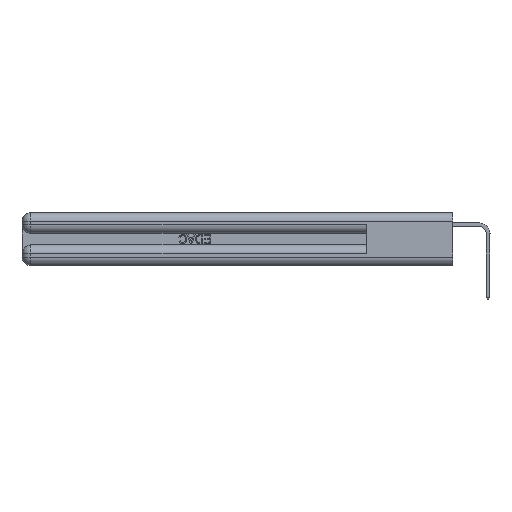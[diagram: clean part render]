
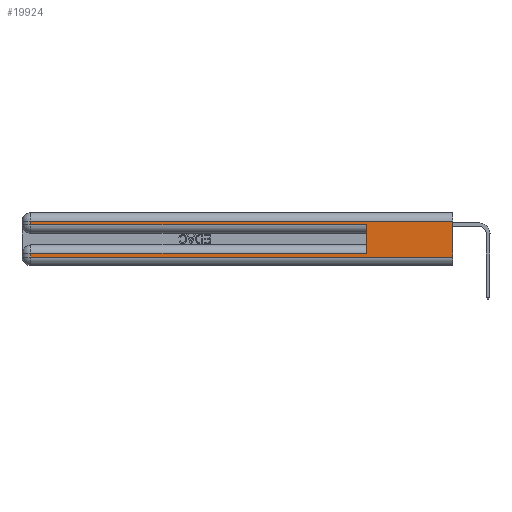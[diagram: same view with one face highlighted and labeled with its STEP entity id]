
A CAD part, left-side view. The second image highlights one B-rep face of the part: STEP entity #19924.
In plain terms, the highlighted planar face has unit normal (-1, 0, 0).
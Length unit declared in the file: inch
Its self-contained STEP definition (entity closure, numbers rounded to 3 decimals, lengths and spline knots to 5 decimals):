
#192 = VERTEX_POINT ( 'NONE', #7704 ) ;
#294 = DIRECTION ( 'NONE',  ( 0., -1., 0. ) ) ;
#431 = ORIENTED_EDGE ( 'NONE', *, *, #45958, .T. ) ;
#3605 = LINE ( 'NONE', #41046, #41292 ) ;
#4216 = CARTESIAN_POINT ( 'NONE',  ( 0., 2.94, 0.31 ) ) ;
#6360 = CARTESIAN_POINT ( 'NONE',  ( 0., 2.94, 0.37 ) ) ;
#6785 = EDGE_CURVE ( 'NONE', #33862, #33027, #36483, .T. ) ;
#7072 = VECTOR ( 'NONE', #30509, 39.37008 ) ;
#7704 = CARTESIAN_POINT ( 'NONE',  ( 0., 0.6, 0.085 ) ) ;
#7809 = CARTESIAN_POINT ( 'NONE',  ( 0., 2.94, 0.285 ) ) ;
#8069 = EDGE_CURVE ( 'NONE', #15839, #33027, #28467, .T. ) ;
#8267 = PLANE ( 'NONE',  #28253 ) ;
#11405 = FACE_OUTER_BOUND ( 'NONE', #26347, .T. ) ;
#11477 = EDGE_CURVE ( 'NONE', #33862, #34792, #3605, .T. ) ;
#11959 = DIRECTION ( 'NONE',  ( 1., 0., 0. ) ) ;
#12282 = EDGE_CURVE ( 'NONE', #23848, #15839, #26407, .T. ) ;
#12825 = CARTESIAN_POINT ( 'NONE',  ( 0., 2.94, 0.085 ) ) ;
#15839 = VERTEX_POINT ( 'NONE', #47384 ) ;
#17404 = EDGE_CURVE ( 'NONE', #192, #23848, #44761, .T. ) ;
#17557 = DIRECTION ( 'NONE',  ( 0., 0., -1. ) ) ;
#18481 = CARTESIAN_POINT ( 'NONE',  ( 0., 0., 0.06 ) ) ;
#19889 = CARTESIAN_POINT ( 'NONE',  ( 0., 2.94, 0.37 ) ) ;
#19924 = ADVANCED_FACE ( 'NONE', ( #11405 ), #8267, .F. ) ;
#20676 = ORIENTED_EDGE ( 'NONE', *, *, #12282, .T. ) ;
#21058 = VERTEX_POINT ( 'NONE', #7809 ) ;
#21318 = CARTESIAN_POINT ( 'NONE',  ( 0., 0., 0.06 ) ) ;
#21478 = DIRECTION ( 'NONE',  ( 0., -1., 0. ) ) ;
#21936 = EDGE_CURVE ( 'NONE', #192, #43079, #38016, .T. ) ;
#23221 = CARTESIAN_POINT ( 'NONE',  ( 0., 0., 0.085 ) ) ;
#23436 = DIRECTION ( 'NONE',  ( 0., 0., -1. ) ) ;
#23437 = ORIENTED_EDGE ( 'NONE', *, *, #28174, .T. ) ;
#23848 = VERTEX_POINT ( 'NONE', #12825 ) ;
#24552 = DIRECTION ( 'NONE',  ( 0., 0., 1. ) ) ;
#25631 = LINE ( 'NONE', #19889, #26745 ) ;
#26347 = EDGE_LOOP ( 'NONE', ( #36931, #46197, #23437, #431, #42446, #27129, #20676, #36000 ) ) ;
#26407 = LINE ( 'NONE', #6360, #44652 ) ;
#26550 = DIRECTION ( 'NONE',  ( 0., 1., 0. ) ) ;
#26745 = VECTOR ( 'NONE', #23436, 39.37008 ) ;
#27129 = ORIENTED_EDGE ( 'NONE', *, *, #17404, .T. ) ;
#27294 = VECTOR ( 'NONE', #21478, 39.37008 ) ;
#28174 = EDGE_CURVE ( 'NONE', #34792, #21058, #25631, .T. ) ;
#28253 = AXIS2_PLACEMENT_3D ( 'NONE', #33844, #11959, #37500 ) ;
#28329 = VECTOR ( 'NONE', #24552, 39.37008 ) ;
#28452 = VECTOR ( 'NONE', #294, 39.37008 ) ;
#28467 = LINE ( 'NONE', #21318, #27294 ) ;
#29569 = LINE ( 'NONE', #44083, #28452 ) ;
#30509 = DIRECTION ( 'NONE',  ( 0., 1., 0. ) ) ;
#33027 = VERTEX_POINT ( 'NONE', #18481 ) ;
#33844 = CARTESIAN_POINT ( 'NONE',  ( 0., 0., 0.37 ) ) ;
#33862 = VERTEX_POINT ( 'NONE', #35009 ) ;
#34792 = VERTEX_POINT ( 'NONE', #4216 ) ;
#35009 = CARTESIAN_POINT ( 'NONE',  ( 0., 0., 0.31 ) ) ;
#35538 = DIRECTION ( 'NONE',  ( 0., 0., -1. ) ) ;
#36000 = ORIENTED_EDGE ( 'NONE', *, *, #8069, .T. ) ;
#36483 = LINE ( 'NONE', #46371, #46183 ) ;
#36931 = ORIENTED_EDGE ( 'NONE', *, *, #6785, .F. ) ;
#37500 = DIRECTION ( 'NONE',  ( 0., 0., -1. ) ) ;
#38016 = LINE ( 'NONE', #39034, #28329 ) ;
#39034 = CARTESIAN_POINT ( 'NONE',  ( 0., 0.6, 0.145 ) ) ;
#41046 = CARTESIAN_POINT ( 'NONE',  ( 0., 0., 0.31 ) ) ;
#41292 = VECTOR ( 'NONE', #26550, 39.37008 ) ;
#42446 = ORIENTED_EDGE ( 'NONE', *, *, #21936, .F. ) ;
#43009 = CARTESIAN_POINT ( 'NONE',  ( 0., 0.6, 0.285 ) ) ;
#43079 = VERTEX_POINT ( 'NONE', #43009 ) ;
#44083 = CARTESIAN_POINT ( 'NONE',  ( 0., 0., 0.285 ) ) ;
#44652 = VECTOR ( 'NONE', #17557, 39.37008 ) ;
#44761 = LINE ( 'NONE', #23221, #7072 ) ;
#45958 = EDGE_CURVE ( 'NONE', #21058, #43079, #29569, .T. ) ;
#46183 = VECTOR ( 'NONE', #35538, 39.37008 ) ;
#46197 = ORIENTED_EDGE ( 'NONE', *, *, #11477, .T. ) ;
#46371 = CARTESIAN_POINT ( 'NONE',  ( 0., 0., 0.37 ) ) ;
#47384 = CARTESIAN_POINT ( 'NONE',  ( 0., 2.94, 0.06 ) ) ;
